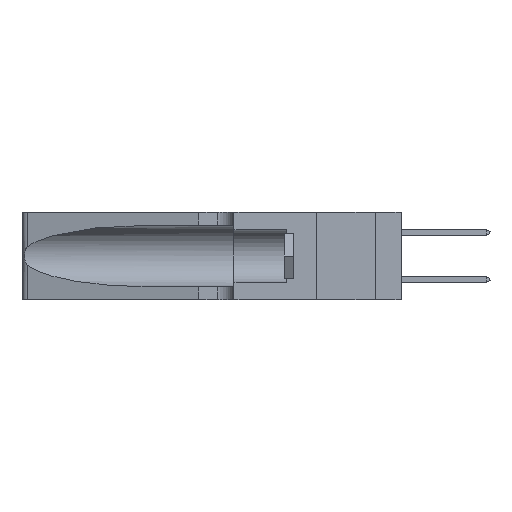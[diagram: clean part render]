
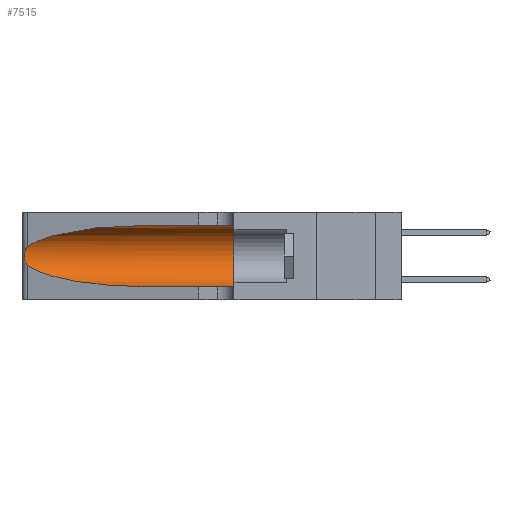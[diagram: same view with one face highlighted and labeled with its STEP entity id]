
A CAD part, left-side view. The second image highlights one B-rep face of the part: STEP entity #7515.
In plain terms, the highlighted cylindrical face has radius 3.308 mm (diameter 6.617 mm), a partial arc.
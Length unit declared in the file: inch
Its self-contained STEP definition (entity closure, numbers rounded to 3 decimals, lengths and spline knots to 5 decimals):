
#734 =( BOUNDED_CURVE ( )  B_SPLINE_CURVE ( 3, ( #5184, #13015, #18774, #7213 ),
 .UNSPECIFIED., .F., .F. ) 
 B_SPLINE_CURVE_WITH_KNOTS ( ( 4, 4 ),
 ( 1.5708, 2.84003 ),
 .UNSPECIFIED. ) 
 CURVE ( )  GEOMETRIC_REPRESENTATION_ITEM ( )  RATIONAL_B_SPLINE_CURVE ( ( 1., 0.87, 0.87, 1. ) ) 
 REPRESENTATION_ITEM ( '' )  );
#1014 = VERTEX_POINT ( 'NONE', #13856 ) ;
#1661 = LINE ( 'NONE', #5587, #22147 ) ;
#1813 = CARTESIAN_POINT ( 'NONE',  ( 0.26075, 1.23896, 0.19203 ) ) ;
#3508 = CARTESIAN_POINT ( 'NONE',  ( 0.1305, 0.35, 0.31525 ) ) ;
#3716 = CARTESIAN_POINT ( 'NONE',  ( 0.25555, 1.22994, 0.2215 ) ) ;
#3796 = CARTESIAN_POINT ( 'NONE',  ( 0.26017, 1.23833, 0.17102 ) ) ;
#4094 = ORIENTED_EDGE ( 'NONE', *, *, #13375, .T. ) ;
#4430 = ORIENTED_EDGE ( 'NONE', *, *, #18386, .T. ) ;
#4661 = ORIENTED_EDGE ( 'NONE', *, *, #11744, .T. ) ;
#4941 = ORIENTED_EDGE ( 'NONE', *, *, #17320, .T. ) ;
#5140 = EDGE_CURVE ( 'NONE', #1014, #15064, #1661, .T. ) ;
#5184 = CARTESIAN_POINT ( 'NONE',  ( 0.1305, 0.72297, 0.31525 ) ) ;
#5204 = ORIENTED_EDGE ( 'NONE', *, *, #10946, .F. ) ;
#5272 = CARTESIAN_POINT ( 'NONE',  ( 0.25487, 1.22718, 0.14631 ) ) ;
#5302 =( BOUNDED_CURVE ( )  B_SPLINE_CURVE ( 3, ( #14101, #23495, #17844, #16028 ),
 .UNSPECIFIED., .F., .T. ) 
 B_SPLINE_CURVE_WITH_KNOTS ( ( 4, 4 ),
 ( 3.44316, 4.71239 ),
 .UNSPECIFIED. ) 
 CURVE ( )  GEOMETRIC_REPRESENTATION_ITEM ( )  RATIONAL_B_SPLINE_CURVE ( ( 1., 0.87, 0.87, 1. ) ) 
 REPRESENTATION_ITEM ( '' )  );
#5343 = ORIENTED_EDGE ( 'NONE', *, *, #5140, .F. ) ;
#5587 = CARTESIAN_POINT ( 'NONE',  ( 0.1305, 1.61858, 0.31525 ) ) ;
#5751 = CARTESIAN_POINT ( 'NONE',  ( 0.25789, 1.23486, 0.15765 ) ) ;
#6324 = CIRCLE ( 'NONE', #12999, 0.13025 ) ;
#7213 = CARTESIAN_POINT ( 'NONE',  ( 0.25487, 1.22718, 0.22369 ) ) ;
#7509 = DIRECTION ( 'NONE',  ( 0., -1., 0. ) ) ;
#7515 = ADVANCED_FACE ( 'NONE', ( #9207 ), #18857, .F. ) ;
#7683 = CARTESIAN_POINT ( 'NONE',  ( 0.25555, 1.22993, 0.14849 ) ) ;
#7780 = VERTEX_POINT ( 'NONE', #9618 ) ;
#8764 = CARTESIAN_POINT ( 'NONE',  ( 0.1305, 1.61858, 0.185 ) ) ;
#9174 = CARTESIAN_POINT ( 'NONE',  ( 0.1305, 0.35, 0.05475 ) ) ;
#9207 = FACE_OUTER_BOUND ( 'NONE', #16163, .T. ) ;
#9618 = CARTESIAN_POINT ( 'NONE',  ( 0.25487, 1.22718, 0.22369 ) ) ;
#10745 = DIRECTION ( 'NONE',  ( 0., -1., 0. ) ) ;
#10946 = EDGE_CURVE ( 'NONE', #15064, #11378, #6324, .T. ) ;
#11378 = VERTEX_POINT ( 'NONE', #9174 ) ;
#11510 = DIRECTION ( 'NONE',  ( 0., 1., 0. ) ) ;
#11532 = CARTESIAN_POINT ( 'NONE',  ( 0.25787, 1.23484, 0.2124 ) ) ;
#11744 = EDGE_CURVE ( 'NONE', #24105, #17570, #5302, .T. ) ;
#12470 = B_SPLINE_CURVE_WITH_KNOTS ( 'NONE', 3,
 ( #19151, #3716, #22903, #11532, #24794, #13497, #1813, #15437, #3796, #17358, #5751, #19230, #7683, #21099 ),
 .UNSPECIFIED., .F., .F.,
 ( 4, 2, 2, 2, 2, 2, 4 ),
 ( 0., 0.00027, 0.00053, 0.00107, 0.0016, 0.00187, 0.00214 ),
 .UNSPECIFIED. ) ;
#12647 = LINE ( 'NONE', #23767, #22713 ) ;
#12999 = AXIS2_PLACEMENT_3D ( 'NONE', #22879, #11510, #24773 ) ;
#13015 = CARTESIAN_POINT ( 'NONE',  ( 0.18966, 0.96281, 0.31525 ) ) ;
#13375 = EDGE_CURVE ( 'NONE', #1014, #7780, #734, .T. ) ;
#13497 = CARTESIAN_POINT ( 'NONE',  ( 0.26018, 1.23835, 0.19895 ) ) ;
#13595 = AXIS2_PLACEMENT_3D ( 'NONE', #8764, #10745, #16522 ) ;
#13856 = CARTESIAN_POINT ( 'NONE',  ( 0.1305, 0.72297, 0.31525 ) ) ;
#14101 = CARTESIAN_POINT ( 'NONE',  ( 0.25487, 1.22718, 0.14631 ) ) ;
#15064 = VERTEX_POINT ( 'NONE', #3508 ) ;
#15437 = CARTESIAN_POINT ( 'NONE',  ( 0.26075, 1.23896, 0.178 ) ) ;
#16028 = CARTESIAN_POINT ( 'NONE',  ( 0.1305, 0.72297, 0.05475 ) ) ;
#16163 = EDGE_LOOP ( 'NONE', ( #4094, #4430, #4661, #4941, #5204, #5343 ) ) ;
#16236 = DIRECTION ( 'NONE',  ( 0., -1., 0. ) ) ;
#16522 = DIRECTION ( 'NONE',  ( 0., 0., -1. ) ) ;
#17320 = EDGE_CURVE ( 'NONE', #17570, #11378, #12647, .T. ) ;
#17358 = CARTESIAN_POINT ( 'NONE',  ( 0.25856, 1.23593, 0.16098 ) ) ;
#17570 = VERTEX_POINT ( 'NONE', #24506 ) ;
#17844 = CARTESIAN_POINT ( 'NONE',  ( 0.18966, 0.96281, 0.05475 ) ) ;
#18386 = EDGE_CURVE ( 'NONE', #7780, #24105, #12470, .T. ) ;
#18774 = CARTESIAN_POINT ( 'NONE',  ( 0.2373, 1.15595, 0.28018 ) ) ;
#18857 = CYLINDRICAL_SURFACE ( 'NONE', #13595, 0.13025 ) ;
#19151 = CARTESIAN_POINT ( 'NONE',  ( 0.25487, 1.22718, 0.22369 ) ) ;
#19230 = CARTESIAN_POINT ( 'NONE',  ( 0.25639, 1.23186, 0.15144 ) ) ;
#21099 = CARTESIAN_POINT ( 'NONE',  ( 0.25487, 1.22718, 0.14631 ) ) ;
#22147 = VECTOR ( 'NONE', #7509, 39.37008 ) ;
#22713 = VECTOR ( 'NONE', #16236, 39.37008 ) ;
#22879 = CARTESIAN_POINT ( 'NONE',  ( 0.1305, 0.35, 0.185 ) ) ;
#22903 = CARTESIAN_POINT ( 'NONE',  ( 0.25639, 1.23184, 0.21858 ) ) ;
#23495 = CARTESIAN_POINT ( 'NONE',  ( 0.2373, 1.15595, 0.08982 ) ) ;
#23767 = CARTESIAN_POINT ( 'NONE',  ( 0.1305, 1.61858, 0.05475 ) ) ;
#24105 = VERTEX_POINT ( 'NONE', #5272 ) ;
#24506 = CARTESIAN_POINT ( 'NONE',  ( 0.1305, 0.72297, 0.05475 ) ) ;
#24773 = DIRECTION ( 'NONE',  ( 0., 0., 1. ) ) ;
#24794 = CARTESIAN_POINT ( 'NONE',  ( 0.25854, 1.2359, 0.20912 ) ) ;
